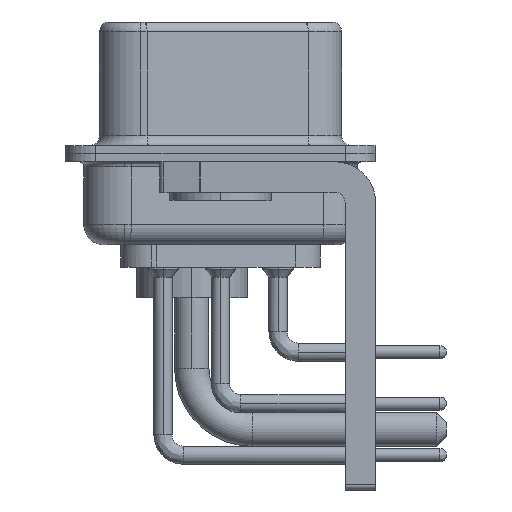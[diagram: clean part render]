
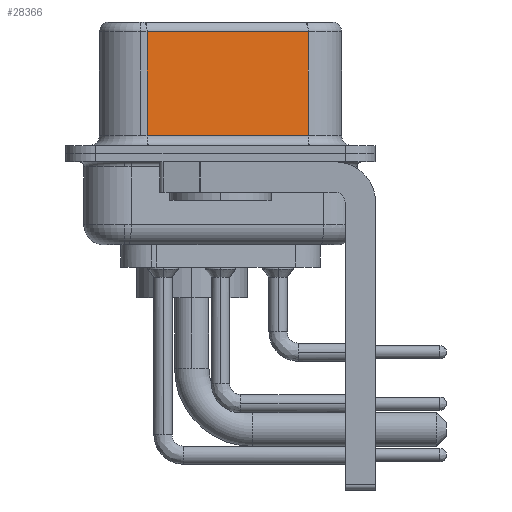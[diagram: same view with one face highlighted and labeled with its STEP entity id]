
A CAD part, left-side view. The second image highlights one B-rep face of the part: STEP entity #28366.
In plain terms, the highlighted planar face has unit normal (-0.985, -0.174, 0).
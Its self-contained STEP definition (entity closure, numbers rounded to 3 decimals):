
#553 = VERTEX_POINT ( 'NONE', #31299 ) ;
#1449 = EDGE_CURVE ( 'NONE', #36637, #11016, #3033, .T. ) ;
#1547 = VERTEX_POINT ( 'NONE', #7828 ) ;
#2199 = VECTOR ( 'NONE', #33334, 1000. ) ;
#2958 = CARTESIAN_POINT ( 'NONE',  ( 3.73, 3.628, 6.52 ) ) ;
#3033 = LINE ( 'NONE', #18633, #2199 ) ;
#3822 = FACE_OUTER_BOUND ( 'NONE', #16324, .T. ) ;
#7828 = CARTESIAN_POINT ( 'NONE',  ( 3.73, 3.628, 0.9 ) ) ;
#9387 = ORIENTED_EDGE ( 'NONE', *, *, #11454, .T. ) ;
#10193 = CARTESIAN_POINT ( 'NONE',  ( 5.132, -4.322, 6.52 ) ) ;
#10956 = EDGE_CURVE ( 'NONE', #1547, #11016, #11311, .T. ) ;
#11016 = VERTEX_POINT ( 'NONE', #17292 ) ;
#11311 = LINE ( 'NONE', #12053, #15811 ) ;
#11454 = EDGE_CURVE ( 'NONE', #553, #1547, #32329, .T. ) ;
#12053 = CARTESIAN_POINT ( 'NONE',  ( 5.132, -4.322, 0.9 ) ) ;
#12224 = ORIENTED_EDGE ( 'NONE', *, *, #10956, .T. ) ;
#13867 = CARTESIAN_POINT ( 'NONE',  ( 5.132, -4.322, 6.02 ) ) ;
#15598 = PLANE ( 'NONE',  #37973 ) ;
#15762 = VECTOR ( 'NONE', #23246, 1000. ) ;
#15811 = VECTOR ( 'NONE', #26002, 1000. ) ;
#15986 = DIRECTION ( 'NONE',  ( 0.985, 0.174, 0. ) ) ;
#16324 = EDGE_LOOP ( 'NONE', ( #36207, #32343, #9387, #12224 ) ) ;
#17292 = CARTESIAN_POINT ( 'NONE',  ( 5.132, -4.322, 0.9 ) ) ;
#18633 = CARTESIAN_POINT ( 'NONE',  ( 5.132, -4.322, 6.52 ) ) ;
#22766 = DIRECTION ( 'NONE',  ( -0.174, 0.985, 0. ) ) ;
#23086 = VECTOR ( 'NONE', #22766, 1000. ) ;
#23246 = DIRECTION ( 'NONE',  ( 0., 0., -1. ) ) ;
#24877 = DIRECTION ( 'NONE',  ( -0.174, 0.985, 0. ) ) ;
#25670 = EDGE_CURVE ( 'NONE', #36637, #553, #27991, .T. ) ;
#26002 = DIRECTION ( 'NONE',  ( 0.174, -0.985, 0. ) ) ;
#27991 = LINE ( 'NONE', #13867, #23086 ) ;
#28366 = ADVANCED_FACE ( 'NONE', ( #3822 ), #15598, .F. ) ;
#30954 = CARTESIAN_POINT ( 'NONE',  ( 5.132, -4.322, 6.02 ) ) ;
#31299 = CARTESIAN_POINT ( 'NONE',  ( 3.73, 3.628, 6.02 ) ) ;
#32329 = LINE ( 'NONE', #2958, #15762 ) ;
#32343 = ORIENTED_EDGE ( 'NONE', *, *, #25670, .T. ) ;
#33334 = DIRECTION ( 'NONE',  ( 0., 0., -1. ) ) ;
#36207 = ORIENTED_EDGE ( 'NONE', *, *, #1449, .F. ) ;
#36637 = VERTEX_POINT ( 'NONE', #30954 ) ;
#37973 = AXIS2_PLACEMENT_3D ( 'NONE', #10193, #15986, #24877 ) ;
